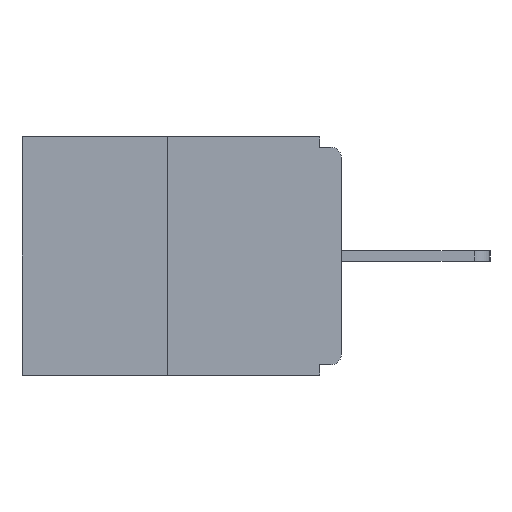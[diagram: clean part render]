
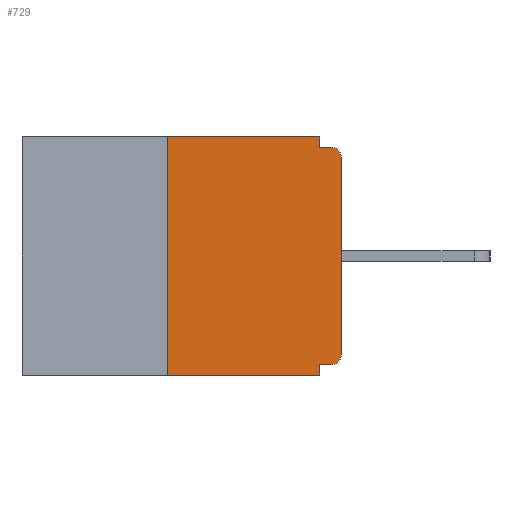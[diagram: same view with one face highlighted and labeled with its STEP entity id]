
A CAD part, left-side view. The second image highlights one B-rep face of the part: STEP entity #729.
In plain terms, the highlighted planar face has unit normal (-1, 0, 0).
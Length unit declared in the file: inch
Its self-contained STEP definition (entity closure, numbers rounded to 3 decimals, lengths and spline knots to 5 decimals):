
#247 = AXIS2_PLACEMENT_3D ( 'NONE', #22942, #10270, #8015 ) ;
#426 = EDGE_CURVE ( 'NONE', #14610, #18366, #7664, .T. ) ;
#711 = CARTESIAN_POINT ( 'NONE',  ( 0., 0.031, 0. ) ) ;
#729 = ADVANCED_FACE ( 'NONE', ( #19272 ), #8461, .F. ) ;
#856 = VECTOR ( 'NONE', #1373, 39.37008 ) ;
#973 = VECTOR ( 'NONE', #8598, 39.37008 ) ;
#1373 = DIRECTION ( 'NONE',  ( 0., -1., 0. ) ) ;
#2646 = CARTESIAN_POINT ( 'NONE',  ( 0., 0.015, -0.313 ) ) ;
#3011 = ORIENTED_EDGE ( 'NONE', *, *, #18927, .F. ) ;
#3042 = CARTESIAN_POINT ( 'NONE',  ( 0., 0.46, -0.343 ) ) ;
#3087 = LINE ( 'NONE', #15411, #5564 ) ;
#3405 = VECTOR ( 'NONE', #20621, 39.37008 ) ;
#3649 = DIRECTION ( 'NONE',  ( -1., 0., 0. ) ) ;
#3885 = DIRECTION ( 'NONE',  ( 0., 1., 0. ) ) ;
#4181 = VERTEX_POINT ( 'NONE', #8234 ) ;
#4252 = DIRECTION ( 'NONE',  ( 0., 0., -1. ) ) ;
#4416 = DIRECTION ( 'NONE',  ( -1., 0., 0. ) ) ;
#4774 = VECTOR ( 'NONE', #19463, 39.37008 ) ;
#5026 = CARTESIAN_POINT ( 'NONE',  ( 0., 0.25, 0. ) ) ;
#5361 = CARTESIAN_POINT ( 'NONE',  ( 0., 0.031, 0. ) ) ;
#5562 = CARTESIAN_POINT ( 'NONE',  ( 0., 0.031, -0.328 ) ) ;
#5564 = VECTOR ( 'NONE', #10200, 39.37008 ) ;
#5567 = VERTEX_POINT ( 'NONE', #5026 ) ;
#5605 = AXIS2_PLACEMENT_3D ( 'NONE', #16557, #3649, #19866 ) ;
#5635 = ORIENTED_EDGE ( 'NONE', *, *, #16463, .T. ) ;
#5969 = VECTOR ( 'NONE', #3885, 39.37008 ) ;
#6208 = CARTESIAN_POINT ( 'NONE',  ( 0., 0., -0.03 ) ) ;
#6787 = LINE ( 'NONE', #12252, #4774 ) ;
#7241 = LINE ( 'NONE', #21710, #22769 ) ;
#7470 = AXIS2_PLACEMENT_3D ( 'NONE', #2646, #4416, #17094 ) ;
#7572 = VERTEX_POINT ( 'NONE', #13363 ) ;
#7664 = LINE ( 'NONE', #11118, #5969 ) ;
#8015 = DIRECTION ( 'NONE',  ( 0., 0., -1. ) ) ;
#8234 = CARTESIAN_POINT ( 'NONE',  ( 0., 0.25, -0.343 ) ) ;
#8461 = PLANE ( 'NONE',  #247 ) ;
#8509 = ORIENTED_EDGE ( 'NONE', *, *, #15133, .F. ) ;
#8598 = DIRECTION ( 'NONE',  ( 0., -1., 0. ) ) ;
#8957 = EDGE_CURVE ( 'NONE', #4181, #7572, #19282, .T. ) ;
#8997 = CIRCLE ( 'NONE', #5605, 0.015 ) ;
#9326 = ORIENTED_EDGE ( 'NONE', *, *, #10740, .T. ) ;
#10043 = EDGE_CURVE ( 'NONE', #18366, #7572, #13269, .T. ) ;
#10109 = CARTESIAN_POINT ( 'NONE',  ( 0., 0.031, -0.015 ) ) ;
#10200 = DIRECTION ( 'NONE',  ( 0., 0., 1. ) ) ;
#10270 = DIRECTION ( 'NONE',  ( 1., 0., 0. ) ) ;
#10612 = VERTEX_POINT ( 'NONE', #17825 ) ;
#10710 = ORIENTED_EDGE ( 'NONE', *, *, #22762, .F. ) ;
#10740 = EDGE_CURVE ( 'NONE', #16024, #12305, #8997, .T. ) ;
#10745 = LINE ( 'NONE', #15954, #856 ) ;
#10877 = CARTESIAN_POINT ( 'NONE',  ( 0., 0.015, -0.328 ) ) ;
#11118 = CARTESIAN_POINT ( 'NONE',  ( 0., 0., -0.328 ) ) ;
#11607 = CARTESIAN_POINT ( 'NONE',  ( 0., 0.031, -0.343 ) ) ;
#11648 = ORIENTED_EDGE ( 'NONE', *, *, #426, .F. ) ;
#11927 = EDGE_CURVE ( 'NONE', #4181, #5567, #3087, .T. ) ;
#12252 = CARTESIAN_POINT ( 'NONE',  ( 0., 0.46, 0. ) ) ;
#12305 = VERTEX_POINT ( 'NONE', #23057 ) ;
#13050 = LINE ( 'NONE', #711, #3405 ) ;
#13269 = LINE ( 'NONE', #11607, #17683 ) ;
#13363 = CARTESIAN_POINT ( 'NONE',  ( 0., 0.031, -0.343 ) ) ;
#14046 = ORIENTED_EDGE ( 'NONE', *, *, #20079, .T. ) ;
#14251 = ORIENTED_EDGE ( 'NONE', *, *, #11927, .F. ) ;
#14610 = VERTEX_POINT ( 'NONE', #10877 ) ;
#15133 = EDGE_CURVE ( 'NONE', #5567, #17772, #6787, .T. ) ;
#15411 = CARTESIAN_POINT ( 'NONE',  ( 0., 0.25, 0. ) ) ;
#15954 = CARTESIAN_POINT ( 'NONE',  ( 0., 0., -0.015 ) ) ;
#16024 = VERTEX_POINT ( 'NONE', #6208 ) ;
#16463 = EDGE_CURVE ( 'NONE', #14610, #10612, #18443, .T. ) ;
#16557 = CARTESIAN_POINT ( 'NONE',  ( 0., 0.015, -0.03 ) ) ;
#16607 = DIRECTION ( 'NONE',  ( 0., 0., 1. ) ) ;
#17094 = DIRECTION ( 'NONE',  ( 0., 0., -1. ) ) ;
#17579 = VERTEX_POINT ( 'NONE', #10109 ) ;
#17683 = VECTOR ( 'NONE', #4252, 39.37008 ) ;
#17772 = VERTEX_POINT ( 'NONE', #5361 ) ;
#17825 = CARTESIAN_POINT ( 'NONE',  ( 0., 0., -0.313 ) ) ;
#17952 = EDGE_LOOP ( 'NONE', ( #8509, #14251, #21618, #22880, #11648, #5635, #14046, #9326, #10710, #3011 ) ) ;
#18366 = VERTEX_POINT ( 'NONE', #5562 ) ;
#18443 = CIRCLE ( 'NONE', #7470, 0.015 ) ;
#18927 = EDGE_CURVE ( 'NONE', #17772, #17579, #13050, .T. ) ;
#19272 = FACE_OUTER_BOUND ( 'NONE', #17952, .T. ) ;
#19282 = LINE ( 'NONE', #3042, #973 ) ;
#19463 = DIRECTION ( 'NONE',  ( 0., -1., 0. ) ) ;
#19866 = DIRECTION ( 'NONE',  ( 0., 0., -1. ) ) ;
#20079 = EDGE_CURVE ( 'NONE', #10612, #16024, #7241, .T. ) ;
#20621 = DIRECTION ( 'NONE',  ( 0., 0., -1. ) ) ;
#21618 = ORIENTED_EDGE ( 'NONE', *, *, #8957, .T. ) ;
#21710 = CARTESIAN_POINT ( 'NONE',  ( 0., 0., 0. ) ) ;
#22762 = EDGE_CURVE ( 'NONE', #17579, #12305, #10745, .T. ) ;
#22769 = VECTOR ( 'NONE', #16607, 39.37008 ) ;
#22880 = ORIENTED_EDGE ( 'NONE', *, *, #10043, .F. ) ;
#22942 = CARTESIAN_POINT ( 'NONE',  ( 0., 0.46, 0. ) ) ;
#23057 = CARTESIAN_POINT ( 'NONE',  ( 0., 0.015, -0.015 ) ) ;
